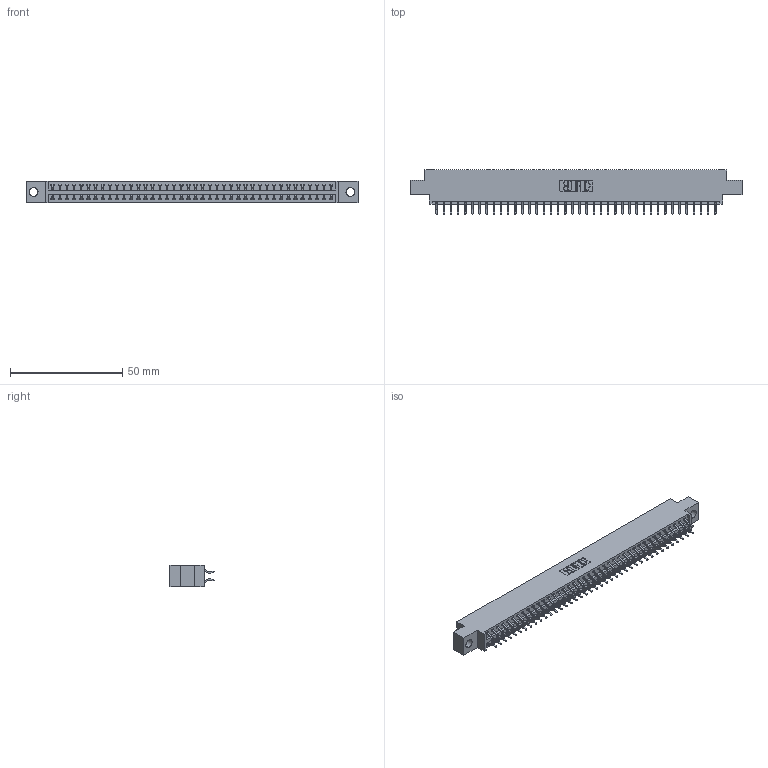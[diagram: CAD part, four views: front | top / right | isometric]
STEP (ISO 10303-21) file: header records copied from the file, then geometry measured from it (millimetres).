
FILE_DESCRIPTION (( 'STEP AP203' ), '1' );
FILE_NAME ('346-080-556-804.STEP', '2022-05-25T16:23:53', ( '' ), ( '' ), 'SwSTEP 2.0', 'SolidWorks 2020', '' );
FILE_SCHEMA (( 'CONFIG_CONTROL_DESIGN' ));
Length unit declared in the file: inch
Products named in the file (3): 345-292-001_556 Tail; 346-080-556-804; 346 Part_0.170 Offset - 0.156 Dia-TH
Assembly tree (81 placements, depth 2):
  346-080-556-804
    346 Part_0.170 Offset - 0.156 Dia-TH
    345-292-001_556 Tail  x80
Bounding box: 147.57 x 19.57 x 9.4 mm (x, y, z)
Volume: 14111 mm3; surface area: 19318.3 mm2
Topology: 81 solids, 81 shells, 4780 faces, 14217 edges, 9370 vertices
Faces by surface type: plane 3214, cylinder 1566
Entity records: 27145 total; most frequent: CARTESIAN_POINT 4498, ORIENTED_EDGE 4418, DIRECTION 4001, EDGE_CURVE 2209, LINE 1909, VECTOR 1909, VERTEX_POINT 1470, AXIS2_PLACEMENT_3D 1046
